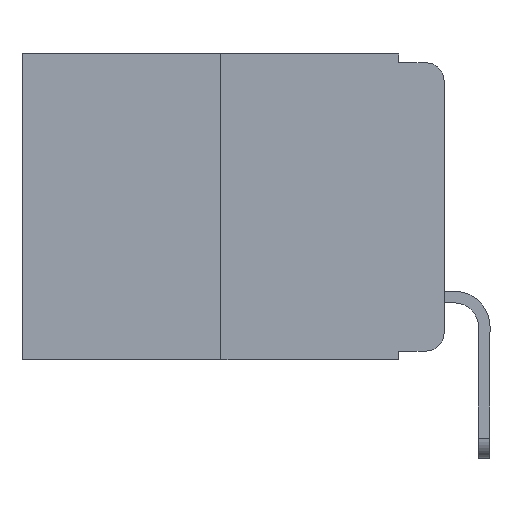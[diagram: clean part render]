
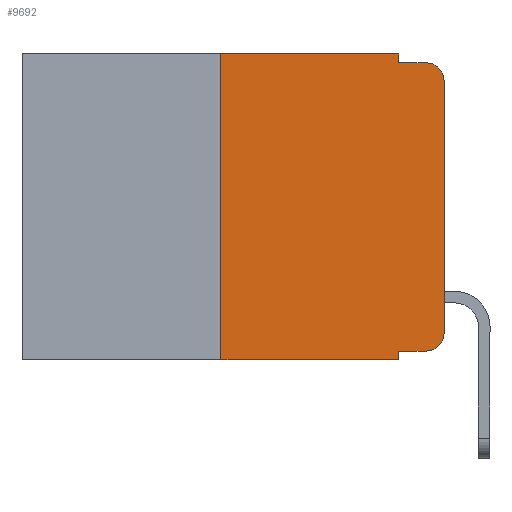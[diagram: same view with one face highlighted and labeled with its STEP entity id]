
A CAD part, left-side view. The second image highlights one B-rep face of the part: STEP entity #9692.
In plain terms, the highlighted planar face has unit normal (-1, 0, 0).
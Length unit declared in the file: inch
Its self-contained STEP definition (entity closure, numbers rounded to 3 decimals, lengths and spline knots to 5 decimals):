
#178 = CARTESIAN_POINT ( 'NONE',  ( 0., 0.25, -0.343 ) ) ;
#284 = VERTEX_POINT ( 'NONE', #4659 ) ;
#428 = PLANE ( 'NONE',  #7665 ) ;
#852 = VECTOR ( 'NONE', #3440, 39.37008 ) ;
#931 = VECTOR ( 'NONE', #14779, 39.37008 ) ;
#1291 = CARTESIAN_POINT ( 'NONE',  ( 0., 0.051, -0.333 ) ) ;
#1474 = ORIENTED_EDGE ( 'NONE', *, *, #18483, .F. ) ;
#1886 = CARTESIAN_POINT ( 'NONE',  ( 0., 0.051, -0.333 ) ) ;
#1994 = VECTOR ( 'NONE', #20080, 39.37008 ) ;
#2411 = DIRECTION ( 'NONE',  ( -1., 0., 0. ) ) ;
#2870 = DIRECTION ( 'NONE',  ( 0., 0., 1. ) ) ;
#2935 = ORIENTED_EDGE ( 'NONE', *, *, #18343, .T. ) ;
#3078 = FACE_OUTER_BOUND ( 'NONE', #3409, .T. ) ;
#3267 = LINE ( 'NONE', #14500, #19607 ) ;
#3355 = EDGE_CURVE ( 'NONE', #18942, #10899, #14382, .T. ) ;
#3409 = EDGE_LOOP ( 'NONE', ( #19799, #2935, #16090, #16573, #21249, #13914, #14396, #1474, #10640, #14894 ) ) ;
#3440 = DIRECTION ( 'NONE',  ( 0., -1., 0. ) ) ;
#3488 = CARTESIAN_POINT ( 'NONE',  ( 0., 0.473, 0. ) ) ;
#3537 = CIRCLE ( 'NONE', #13870, 0.02 ) ;
#3851 = VERTEX_POINT ( 'NONE', #11835 ) ;
#3927 = CARTESIAN_POINT ( 'NONE',  ( 0., 0.051, 0. ) ) ;
#4659 = CARTESIAN_POINT ( 'NONE',  ( 0., 0., -0.313 ) ) ;
#5844 = CARTESIAN_POINT ( 'NONE',  ( 0., 0.473, 0. ) ) ;
#6057 = VERTEX_POINT ( 'NONE', #1886 ) ;
#6441 = CARTESIAN_POINT ( 'NONE',  ( 0., 0.051, 0. ) ) ;
#6962 = CARTESIAN_POINT ( 'NONE',  ( 0., 0.02, -0.313 ) ) ;
#7213 = CARTESIAN_POINT ( 'NONE',  ( 0., 0., 0. ) ) ;
#7529 = DIRECTION ( 'NONE',  ( 0., 0., -1. ) ) ;
#7665 = AXIS2_PLACEMENT_3D ( 'NONE', #5844, #17171, #7529 ) ;
#7827 = CARTESIAN_POINT ( 'NONE',  ( 0., 0.051, -0.01 ) ) ;
#7960 = DIRECTION ( 'NONE',  ( 0., 0., -1. ) ) ;
#8273 = LINE ( 'NONE', #7827, #21081 ) ;
#8650 = DIRECTION ( 'NONE',  ( 0., 0., -1. ) ) ;
#8896 = DIRECTION ( 'NONE',  ( 0., 0., 1. ) ) ;
#9123 = VERTEX_POINT ( 'NONE', #13943 ) ;
#9227 = AXIS2_PLACEMENT_3D ( 'NONE', #12492, #2411, #14107 ) ;
#9621 = LINE ( 'NONE', #1291, #931 ) ;
#9692 = ADVANCED_FACE ( 'NONE', ( #3078 ), #428, .F. ) ;
#10172 = VECTOR ( 'NONE', #13037, 39.37008 ) ;
#10243 = CARTESIAN_POINT ( 'NONE',  ( 0., 0.051, -0.01 ) ) ;
#10591 = CARTESIAN_POINT ( 'NONE',  ( 0., 0.02, -0.01 ) ) ;
#10640 = ORIENTED_EDGE ( 'NONE', *, *, #18515, .T. ) ;
#10693 = LINE ( 'NONE', #6441, #10172 ) ;
#10845 = VERTEX_POINT ( 'NONE', #10591 ) ;
#10899 = VERTEX_POINT ( 'NONE', #3927 ) ;
#11044 = LINE ( 'NONE', #12175, #1994 ) ;
#11607 = VERTEX_POINT ( 'NONE', #178 ) ;
#11835 = CARTESIAN_POINT ( 'NONE',  ( 0., 0., -0.03 ) ) ;
#12175 = CARTESIAN_POINT ( 'NONE',  ( 0., 0.473, -0.343 ) ) ;
#12492 = CARTESIAN_POINT ( 'NONE',  ( 0., 0.02, -0.03 ) ) ;
#13037 = DIRECTION ( 'NONE',  ( 0., 0., -1. ) ) ;
#13870 = AXIS2_PLACEMENT_3D ( 'NONE', #6962, #18268, #8650 ) ;
#13914 = ORIENTED_EDGE ( 'NONE', *, *, #18450, .F. ) ;
#13943 = CARTESIAN_POINT ( 'NONE',  ( 0., 0.02, -0.333 ) ) ;
#14107 = DIRECTION ( 'NONE',  ( 0., 0., -1. ) ) ;
#14382 = LINE ( 'NONE', #3488, #852 ) ;
#14396 = ORIENTED_EDGE ( 'NONE', *, *, #16066, .T. ) ;
#14500 = CARTESIAN_POINT ( 'NONE',  ( 0., 0.25, 0. ) ) ;
#14779 = DIRECTION ( 'NONE',  ( 0., -1., 0. ) ) ;
#14894 = ORIENTED_EDGE ( 'NONE', *, *, #18602, .T. ) ;
#15385 = VERTEX_POINT ( 'NONE', #18419 ) ;
#15903 = LINE ( 'NONE', #17619, #20126 ) ;
#16066 = EDGE_CURVE ( 'NONE', #11607, #15385, #11044, .T. ) ;
#16090 = ORIENTED_EDGE ( 'NONE', *, *, #18415, .F. ) ;
#16168 = VECTOR ( 'NONE', #8896, 39.37008 ) ;
#16445 = CARTESIAN_POINT ( 'NONE',  ( 0., 0.25, 0. ) ) ;
#16573 = ORIENTED_EDGE ( 'NONE', *, *, #18445, .F. ) ;
#16643 = LINE ( 'NONE', #7213, #16168 ) ;
#17171 = DIRECTION ( 'NONE',  ( 1., 0., 0. ) ) ;
#17619 = CARTESIAN_POINT ( 'NONE',  ( 0., 0.051, 0. ) ) ;
#18253 = VERTEX_POINT ( 'NONE', #10243 ) ;
#18268 = DIRECTION ( 'NONE',  ( -1., 0., 0. ) ) ;
#18282 = EDGE_CURVE ( 'NONE', #284, #3851, #16643, .T. ) ;
#18343 = EDGE_CURVE ( 'NONE', #3851, #10845, #18391, .T. ) ;
#18391 = CIRCLE ( 'NONE', #9227, 0.02 ) ;
#18415 = EDGE_CURVE ( 'NONE', #18253, #10845, #8273, .T. ) ;
#18419 = CARTESIAN_POINT ( 'NONE',  ( 0., 0.051, -0.343 ) ) ;
#18445 = EDGE_CURVE ( 'NONE', #10899, #18253, #15903, .T. ) ;
#18450 = EDGE_CURVE ( 'NONE', #11607, #18942, #3267, .T. ) ;
#18483 = EDGE_CURVE ( 'NONE', #6057, #15385, #10693, .T. ) ;
#18515 = EDGE_CURVE ( 'NONE', #6057, #9123, #9621, .T. ) ;
#18602 = EDGE_CURVE ( 'NONE', #9123, #284, #3537, .T. ) ;
#18942 = VERTEX_POINT ( 'NONE', #16445 ) ;
#19126 = DIRECTION ( 'NONE',  ( 0., -1., 0. ) ) ;
#19607 = VECTOR ( 'NONE', #2870, 39.37008 ) ;
#19799 = ORIENTED_EDGE ( 'NONE', *, *, #18282, .T. ) ;
#20080 = DIRECTION ( 'NONE',  ( 0., -1., 0. ) ) ;
#20126 = VECTOR ( 'NONE', #7960, 39.37008 ) ;
#21081 = VECTOR ( 'NONE', #19126, 39.37008 ) ;
#21249 = ORIENTED_EDGE ( 'NONE', *, *, #3355, .F. ) ;
